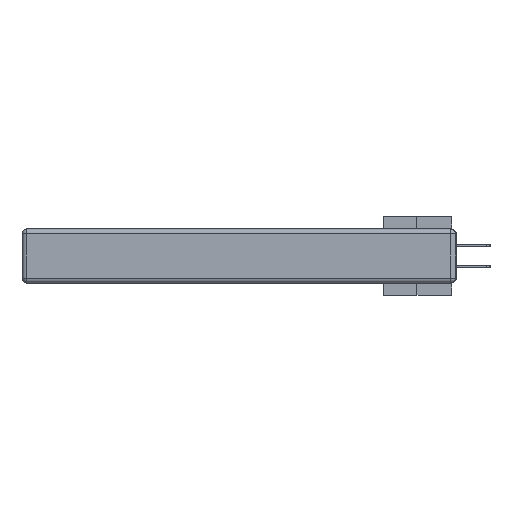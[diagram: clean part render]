
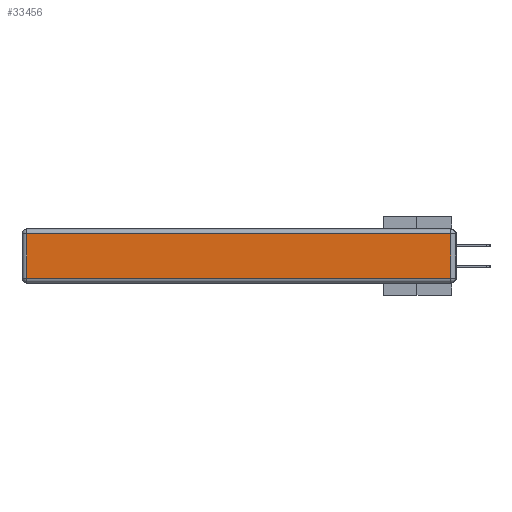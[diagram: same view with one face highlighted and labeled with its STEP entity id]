
A CAD part, left-side view. The second image highlights one B-rep face of the part: STEP entity #33456.
In plain terms, the highlighted planar face has unit normal (-1, 0, 0).
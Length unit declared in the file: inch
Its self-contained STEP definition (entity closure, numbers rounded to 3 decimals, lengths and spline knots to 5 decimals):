
#896 = VERTEX_POINT ( 'NONE', #39977 ) ;
#2033 = DIRECTION ( 'NONE',  ( -1., 0., 0. ) ) ;
#3241 = LINE ( 'NONE', #33751, #20601 ) ;
#4055 = FACE_OUTER_BOUND ( 'NONE', #29141, .T. ) ;
#4176 = VERTEX_POINT ( 'NONE', #6382 ) ;
#5855 = DIRECTION ( 'NONE',  ( 0., -1., 0. ) ) ;
#6382 = CARTESIAN_POINT ( 'NONE',  ( 0., 2.72, -0.03 ) ) ;
#8285 = AXIS2_PLACEMENT_3D ( 'NONE', #21578, #2033, #24869 ) ;
#11578 = LINE ( 'NONE', #41478, #12572 ) ;
#11730 = CARTESIAN_POINT ( 'NONE',  ( 0., 2.72, -0.313 ) ) ;
#12046 = CARTESIAN_POINT ( 'NONE',  ( 0., 2.72, -0.343 ) ) ;
#12572 = VECTOR ( 'NONE', #5855, 39.37008 ) ;
#14369 = DIRECTION ( 'NONE',  ( 0., 0., 1. ) ) ;
#17007 = ORIENTED_EDGE ( 'NONE', *, *, #34563, .T. ) ;
#18759 = DIRECTION ( 'NONE',  ( 0., 0., -1. ) ) ;
#20601 = VECTOR ( 'NONE', #14369, 39.37008 ) ;
#20808 = CARTESIAN_POINT ( 'NONE',  ( 0., 2.75, -0.03 ) ) ;
#21578 = CARTESIAN_POINT ( 'NONE',  ( 0., 0., -0.343 ) ) ;
#24332 = EDGE_CURVE ( 'NONE', #39620, #896, #3241, .T. ) ;
#24869 = DIRECTION ( 'NONE',  ( 0., 0., 1. ) ) ;
#25797 = VECTOR ( 'NONE', #30808, 39.37008 ) ;
#29141 = EDGE_LOOP ( 'NONE', ( #17007, #39459, #29727, #36991 ) ) ;
#29727 = ORIENTED_EDGE ( 'NONE', *, *, #36603, .T. ) ;
#30479 = CARTESIAN_POINT ( 'NONE',  ( 0., 0.03, -0.313 ) ) ;
#30808 = DIRECTION ( 'NONE',  ( 0., 1., 0. ) ) ;
#32461 = LINE ( 'NONE', #20808, #25797 ) ;
#33456 = ADVANCED_FACE ( 'NONE', ( #4055 ), #41761, .T. ) ;
#33751 = CARTESIAN_POINT ( 'NONE',  ( 0., 0.03, -0.343 ) ) ;
#34563 = EDGE_CURVE ( 'NONE', #36769, #39620, #11578, .T. ) ;
#36245 = LINE ( 'NONE', #12046, #38305 ) ;
#36603 = EDGE_CURVE ( 'NONE', #896, #4176, #32461, .T. ) ;
#36769 = VERTEX_POINT ( 'NONE', #11730 ) ;
#36991 = ORIENTED_EDGE ( 'NONE', *, *, #41491, .T. ) ;
#38305 = VECTOR ( 'NONE', #18759, 39.37008 ) ;
#39459 = ORIENTED_EDGE ( 'NONE', *, *, #24332, .T. ) ;
#39620 = VERTEX_POINT ( 'NONE', #30479 ) ;
#39977 = CARTESIAN_POINT ( 'NONE',  ( 0., 0.03, -0.03 ) ) ;
#41478 = CARTESIAN_POINT ( 'NONE',  ( 0., 0., -0.313 ) ) ;
#41491 = EDGE_CURVE ( 'NONE', #4176, #36769, #36245, .T. ) ;
#41761 = PLANE ( 'NONE',  #8285 ) ;
